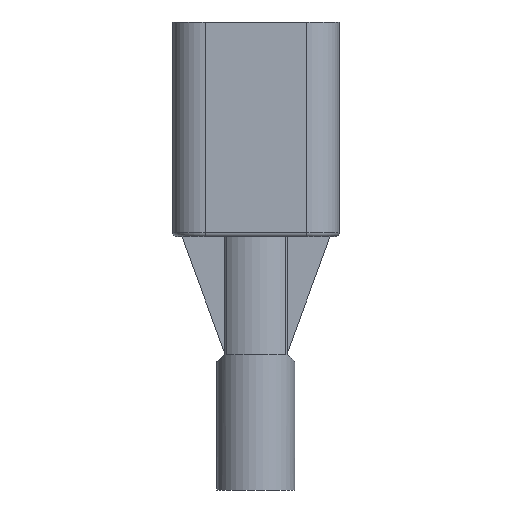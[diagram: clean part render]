
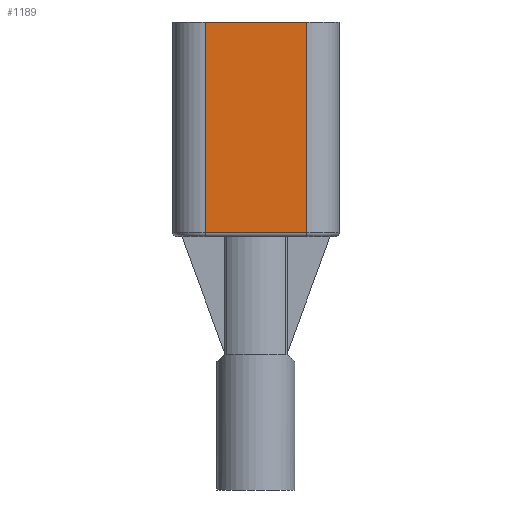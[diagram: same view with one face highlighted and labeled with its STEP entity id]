
A CAD part, front view. The second image highlights one B-rep face of the part: STEP entity #1189.
In plain terms, the highlighted planar face has unit normal (0, -1, 0).
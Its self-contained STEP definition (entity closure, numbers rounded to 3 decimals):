
#50 = VERTEX_POINT ( 'NONE', #2274 ) ;
#135 = ORIENTED_EDGE ( 'NONE', *, *, #1686, .T. ) ;
#309 = DIRECTION ( 'NONE',  ( 0., 0., -1. ) ) ;
#546 = CARTESIAN_POINT ( 'NONE',  ( -3.9, 0., 16.5 ) ) ;
#557 = AXIS2_PLACEMENT_3D ( 'NONE', #546, #4270, #2518 ) ;
#814 = LINE ( 'NONE', #1039, #1760 ) ;
#856 = FACE_OUTER_BOUND ( 'NONE', #2196, .T. ) ;
#916 = VECTOR ( 'NONE', #2232, 1000. ) ;
#979 = LINE ( 'NONE', #1715, #3001 ) ;
#1039 = CARTESIAN_POINT ( 'NONE',  ( 3.9, 0., 16.5 ) ) ;
#1052 = EDGE_CURVE ( 'NONE', #3252, #50, #814, .T. ) ;
#1126 = ORIENTED_EDGE ( 'NONE', *, *, #1052, .F. ) ;
#1133 = VERTEX_POINT ( 'NONE', #1450 ) ;
#1140 = LINE ( 'NONE', #4118, #2041 ) ;
#1189 = ADVANCED_FACE ( 'NONE', ( #856 ), #3199, .F. ) ;
#1224 = EDGE_CURVE ( 'NONE', #1133, #3252, #2898, .T. ) ;
#1321 = EDGE_CURVE ( 'NONE', #3711, #50, #1140, .T. ) ;
#1450 = CARTESIAN_POINT ( 'NONE',  ( -3.9, 0., 16.5 ) ) ;
#1479 = ORIENTED_EDGE ( 'NONE', *, *, #1321, .T. ) ;
#1652 = CARTESIAN_POINT ( 'NONE',  ( -3.9, 0., 0.3 ) ) ;
#1680 = CARTESIAN_POINT ( 'NONE',  ( 3.9, 0., 16.5 ) ) ;
#1686 = EDGE_CURVE ( 'NONE', #1133, #3711, #979, .T. ) ;
#1715 = CARTESIAN_POINT ( 'NONE',  ( -3.9, 0., 16.5 ) ) ;
#1760 = VECTOR ( 'NONE', #2166, 1000. ) ;
#2041 = VECTOR ( 'NONE', #2510, 1000. ) ;
#2166 = DIRECTION ( 'NONE',  ( 0., 0., -1. ) ) ;
#2196 = EDGE_LOOP ( 'NONE', ( #1126, #2731, #135, #1479 ) ) ;
#2212 = CARTESIAN_POINT ( 'NONE',  ( -3.9, 0., 16.5 ) ) ;
#2232 = DIRECTION ( 'NONE',  ( 1., 0., 0. ) ) ;
#2274 = CARTESIAN_POINT ( 'NONE',  ( 3.9, 0., 0.3 ) ) ;
#2510 = DIRECTION ( 'NONE',  ( 1., 0., 0. ) ) ;
#2518 = DIRECTION ( 'NONE',  ( -1., 0., 0. ) ) ;
#2731 = ORIENTED_EDGE ( 'NONE', *, *, #1224, .F. ) ;
#2898 = LINE ( 'NONE', #2212, #916 ) ;
#3001 = VECTOR ( 'NONE', #309, 1000. ) ;
#3199 = PLANE ( 'NONE',  #557 ) ;
#3252 = VERTEX_POINT ( 'NONE', #1680 ) ;
#3711 = VERTEX_POINT ( 'NONE', #1652 ) ;
#4118 = CARTESIAN_POINT ( 'NONE',  ( -3.9, 0., 0.3 ) ) ;
#4270 = DIRECTION ( 'NONE',  ( 0., 1., 0. ) ) ;
